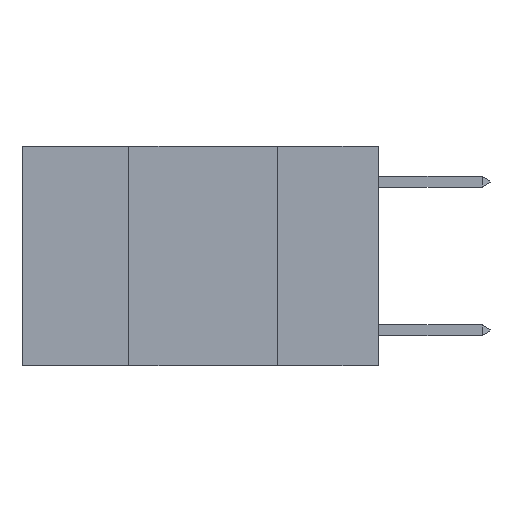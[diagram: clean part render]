
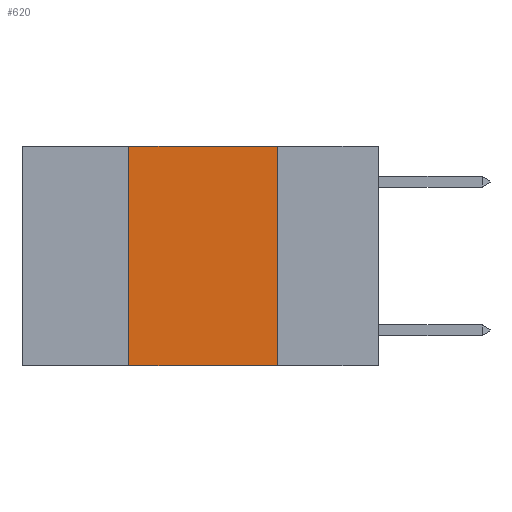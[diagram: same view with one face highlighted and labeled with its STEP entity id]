
A CAD part, left-side view. The second image highlights one B-rep face of the part: STEP entity #620.
In plain terms, the highlighted planar face has unit normal (-1, 0, 0).
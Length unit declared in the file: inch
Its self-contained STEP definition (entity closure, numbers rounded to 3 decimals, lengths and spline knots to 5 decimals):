
#130 = ORIENTED_EDGE ( 'NONE', *, *, #8244, .F. ) ;
#242 = EDGE_CURVE ( 'NONE', #24333, #9493, #4608, .T. ) ;
#620 = ADVANCED_FACE ( 'NONE', ( #6771 ), #14529, .F. ) ;
#857 = DIRECTION ( 'NONE',  ( 0., 0., 1. ) ) ;
#1256 = CARTESIAN_POINT ( 'NONE',  ( 0., 0.17, -0.37 ) ) ;
#1632 = VECTOR ( 'NONE', #857, 39.37008 ) ;
#2639 = DIRECTION ( 'NONE',  ( 0., 0., -1. ) ) ;
#4565 = ORIENTED_EDGE ( 'NONE', *, *, #5489, .T. ) ;
#4608 = LINE ( 'NONE', #8879, #1632 ) ;
#4817 = LINE ( 'NONE', #24467, #24099 ) ;
#5293 = DIRECTION ( 'NONE',  ( 0., -1., 0. ) ) ;
#5489 = EDGE_CURVE ( 'NONE', #24333, #6061, #22878, .T. ) ;
#6061 = VERTEX_POINT ( 'NONE', #1256 ) ;
#6380 = DIRECTION ( 'NONE',  ( 0., -1., 0. ) ) ;
#6771 = FACE_OUTER_BOUND ( 'NONE', #22578, .T. ) ;
#6991 = CARTESIAN_POINT ( 'NONE',  ( 0., 0.17, 0. ) ) ;
#7442 = ORIENTED_EDGE ( 'NONE', *, *, #242, .F. ) ;
#8244 = EDGE_CURVE ( 'NONE', #9493, #18613, #4817, .T. ) ;
#8879 = CARTESIAN_POINT ( 'NONE',  ( 0., 0.42, 0. ) ) ;
#8998 = DIRECTION ( 'NONE',  ( 0., 0., -1. ) ) ;
#9308 = CARTESIAN_POINT ( 'NONE',  ( 0., 0.6, -0.37 ) ) ;
#9486 = VECTOR ( 'NONE', #5293, 39.37008 ) ;
#9493 = VERTEX_POINT ( 'NONE', #14948 ) ;
#10133 = VECTOR ( 'NONE', #8998, 39.37008 ) ;
#10657 = DIRECTION ( 'NONE',  ( 1., 0., 0. ) ) ;
#10931 = LINE ( 'NONE', #12716, #10133 ) ;
#12716 = CARTESIAN_POINT ( 'NONE',  ( 0., 0.17, 0. ) ) ;
#14529 = PLANE ( 'NONE',  #14944 ) ;
#14919 = CARTESIAN_POINT ( 'NONE',  ( 0., 0.6, 0. ) ) ;
#14944 = AXIS2_PLACEMENT_3D ( 'NONE', #14919, #10657, #2639 ) ;
#14948 = CARTESIAN_POINT ( 'NONE',  ( 0., 0.42, 0. ) ) ;
#18613 = VERTEX_POINT ( 'NONE', #6991 ) ;
#21435 = CARTESIAN_POINT ( 'NONE',  ( 0., 0.42, -0.37 ) ) ;
#22578 = EDGE_LOOP ( 'NONE', ( #22741, #130, #7442, #4565 ) ) ;
#22741 = ORIENTED_EDGE ( 'NONE', *, *, #22783, .F. ) ;
#22783 = EDGE_CURVE ( 'NONE', #18613, #6061, #10931, .T. ) ;
#22878 = LINE ( 'NONE', #9308, #9486 ) ;
#24099 = VECTOR ( 'NONE', #6380, 39.37008 ) ;
#24333 = VERTEX_POINT ( 'NONE', #21435 ) ;
#24467 = CARTESIAN_POINT ( 'NONE',  ( 0., 0.6, 0. ) ) ;
